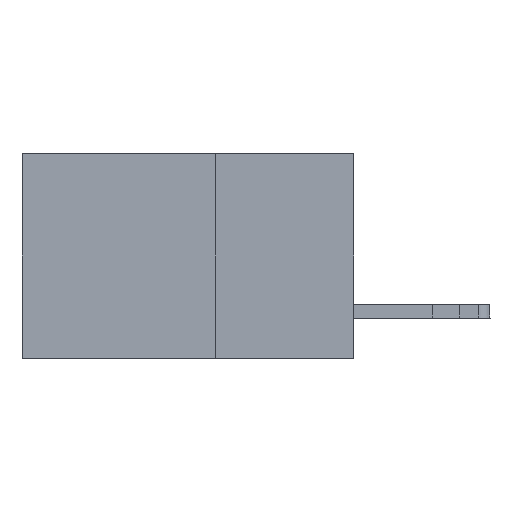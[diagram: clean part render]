
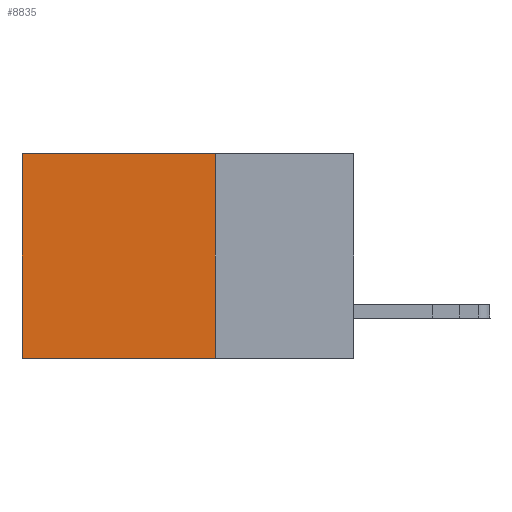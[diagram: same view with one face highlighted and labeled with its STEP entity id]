
A CAD part, left-side view. The second image highlights one B-rep face of the part: STEP entity #8835.
In plain terms, the highlighted planar face has unit normal (-1, 0, 0).
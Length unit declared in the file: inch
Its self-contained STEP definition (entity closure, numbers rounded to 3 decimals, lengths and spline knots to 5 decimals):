
#2385 = DIRECTION ( 'NONE',  ( 0., 0., -1. ) ) ;
#2533 = DIRECTION ( 'NONE',  ( 0., 0., -1. ) ) ;
#3285 = VERTEX_POINT ( 'NONE', #10433 ) ;
#4059 = VERTEX_POINT ( 'NONE', #5922 ) ;
#5408 = LINE ( 'NONE', #15694, #20377 ) ;
#5809 = EDGE_CURVE ( 'NONE', #8701, #4059, #5408, .T. ) ;
#5922 = CARTESIAN_POINT ( 'NONE',  ( 0.2875, 0.6, -0.37 ) ) ;
#6025 = CARTESIAN_POINT ( 'NONE',  ( 0.2875, 0.25, -0.37 ) ) ;
#6424 = LINE ( 'NONE', #31582, #15571 ) ;
#6741 = LINE ( 'NONE', #19236, #32273 ) ;
#7142 = EDGE_LOOP ( 'NONE', ( #10930, #22351, #27446, #21157 ) ) ;
#8549 = DIRECTION ( 'NONE',  ( 0., 1., 0. ) ) ;
#8701 = VERTEX_POINT ( 'NONE', #14224 ) ;
#8835 = ADVANCED_FACE ( 'NONE', ( #15038 ), #15209, .F. ) ;
#9047 = EDGE_CURVE ( 'NONE', #3285, #12421, #6741, .T. ) ;
#10433 = CARTESIAN_POINT ( 'NONE',  ( 0.2875, 0.25, 0. ) ) ;
#10814 = CARTESIAN_POINT ( 'NONE',  ( 0.2875, 0.25, -0.37 ) ) ;
#10930 = ORIENTED_EDGE ( 'NONE', *, *, #5809, .T. ) ;
#12421 = VERTEX_POINT ( 'NONE', #10814 ) ;
#14198 = DIRECTION ( 'NONE',  ( 0., 1., 0. ) ) ;
#14224 = CARTESIAN_POINT ( 'NONE',  ( 0.2875, 0.6, 0. ) ) ;
#14346 = DIRECTION ( 'NONE',  ( 0., 0., -1. ) ) ;
#15038 = FACE_OUTER_BOUND ( 'NONE', #7142, .T. ) ;
#15209 = PLANE ( 'NONE',  #18215 ) ;
#15571 = VECTOR ( 'NONE', #14198, 39.37008 ) ;
#15694 = CARTESIAN_POINT ( 'NONE',  ( 0.2875, 0.6, 0. ) ) ;
#17854 = VECTOR ( 'NONE', #8549, 39.37008 ) ;
#18215 = AXIS2_PLACEMENT_3D ( 'NONE', #25331, #25487, #2385 ) ;
#18675 = EDGE_CURVE ( 'NONE', #12421, #4059, #19010, .T. ) ;
#19010 = LINE ( 'NONE', #6025, #17854 ) ;
#19236 = CARTESIAN_POINT ( 'NONE',  ( 0.2875, 0.25, 0. ) ) ;
#20377 = VECTOR ( 'NONE', #2533, 39.37008 ) ;
#21157 = ORIENTED_EDGE ( 'NONE', *, *, #30688, .T. ) ;
#22351 = ORIENTED_EDGE ( 'NONE', *, *, #18675, .F. ) ;
#25331 = CARTESIAN_POINT ( 'NONE',  ( 0.2875, 0.25, 0. ) ) ;
#25487 = DIRECTION ( 'NONE',  ( 1., 0., 0. ) ) ;
#27446 = ORIENTED_EDGE ( 'NONE', *, *, #9047, .F. ) ;
#30688 = EDGE_CURVE ( 'NONE', #3285, #8701, #6424, .T. ) ;
#31582 = CARTESIAN_POINT ( 'NONE',  ( 0.2875, 0.25, 0. ) ) ;
#32273 = VECTOR ( 'NONE', #14346, 39.37008 ) ;
